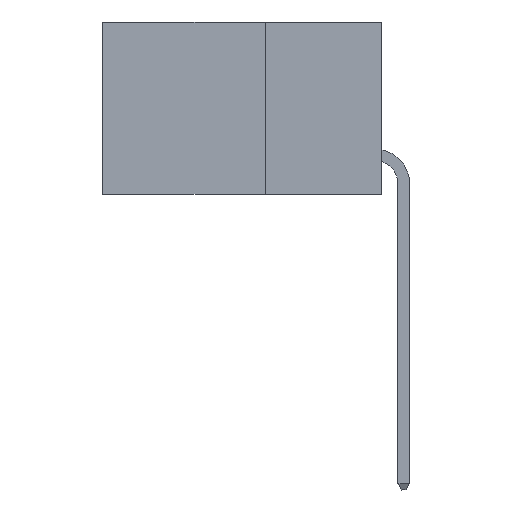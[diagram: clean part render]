
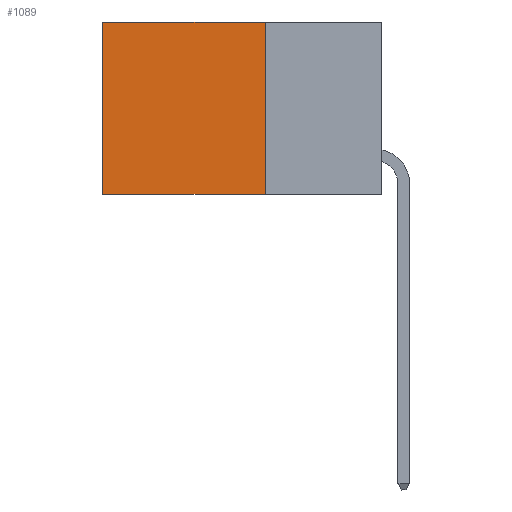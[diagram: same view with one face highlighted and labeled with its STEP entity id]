
A CAD part, left-side view. The second image highlights one B-rep face of the part: STEP entity #1089.
In plain terms, the highlighted planar face has unit normal (-1, 0, 0).
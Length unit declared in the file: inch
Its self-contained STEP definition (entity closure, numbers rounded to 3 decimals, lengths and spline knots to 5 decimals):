
#391 = DIRECTION ( 'NONE',  ( 0., 1., 0. ) ) ;
#1089 = ADVANCED_FACE ( 'NONE', ( #2454 ), #1343, .F. ) ;
#1343 = PLANE ( 'NONE',  #5327 ) ;
#1380 = VERTEX_POINT ( 'NONE', #11196 ) ;
#1478 = CARTESIAN_POINT ( 'NONE',  ( 0.2875, 0.25, 0. ) ) ;
#1891 = EDGE_CURVE ( 'NONE', #3448, #11308, #9385, .T. ) ;
#2344 = ORIENTED_EDGE ( 'NONE', *, *, #2381, .F. ) ;
#2381 = EDGE_CURVE ( 'NONE', #9635, #1380, #6919, .T. ) ;
#2402 = DIRECTION ( 'NONE',  ( 1., 0., 0. ) ) ;
#2454 = FACE_OUTER_BOUND ( 'NONE', #6798, .T. ) ;
#2657 = DIRECTION ( 'NONE',  ( 0., 0., -1. ) ) ;
#3448 = VERTEX_POINT ( 'NONE', #6373 ) ;
#3698 = ORIENTED_EDGE ( 'NONE', *, *, #6172, .T. ) ;
#3722 = CARTESIAN_POINT ( 'NONE',  ( 0.2875, 0.6, 0. ) ) ;
#4251 = DIRECTION ( 'NONE',  ( 0., 1., 0. ) ) ;
#5292 = LINE ( 'NONE', #1478, #11238 ) ;
#5327 = AXIS2_PLACEMENT_3D ( 'NONE', #9189, #2402, #7101 ) ;
#6158 = CARTESIAN_POINT ( 'NONE',  ( 0.2875, 0.25, -0.37 ) ) ;
#6172 = EDGE_CURVE ( 'NONE', #9635, #3448, #5292, .T. ) ;
#6373 = CARTESIAN_POINT ( 'NONE',  ( 0.2875, 0.6, 0. ) ) ;
#6435 = CARTESIAN_POINT ( 'NONE',  ( 0.2875, 0.25, 0. ) ) ;
#6503 = VECTOR ( 'NONE', #391, 39.37008 ) ;
#6702 = ORIENTED_EDGE ( 'NONE', *, *, #7268, .F. ) ;
#6798 = EDGE_LOOP ( 'NONE', ( #12119, #6702, #2344, #3698 ) ) ;
#6919 = LINE ( 'NONE', #6435, #11629 ) ;
#7101 = DIRECTION ( 'NONE',  ( 0., 0., -1. ) ) ;
#7268 = EDGE_CURVE ( 'NONE', #1380, #11308, #8161, .T. ) ;
#7616 = DIRECTION ( 'NONE',  ( 0., 0., -1. ) ) ;
#7692 = VECTOR ( 'NONE', #7616, 39.37008 ) ;
#8161 = LINE ( 'NONE', #6158, #6503 ) ;
#8809 = CARTESIAN_POINT ( 'NONE',  ( 0.2875, 0.6, -0.37 ) ) ;
#9189 = CARTESIAN_POINT ( 'NONE',  ( 0.2875, 0.25, 0. ) ) ;
#9385 = LINE ( 'NONE', #3722, #7692 ) ;
#9635 = VERTEX_POINT ( 'NONE', #10437 ) ;
#10437 = CARTESIAN_POINT ( 'NONE',  ( 0.2875, 0.25, 0. ) ) ;
#11196 = CARTESIAN_POINT ( 'NONE',  ( 0.2875, 0.25, -0.37 ) ) ;
#11238 = VECTOR ( 'NONE', #4251, 39.37008 ) ;
#11308 = VERTEX_POINT ( 'NONE', #8809 ) ;
#11629 = VECTOR ( 'NONE', #2657, 39.37008 ) ;
#12119 = ORIENTED_EDGE ( 'NONE', *, *, #1891, .T. ) ;
